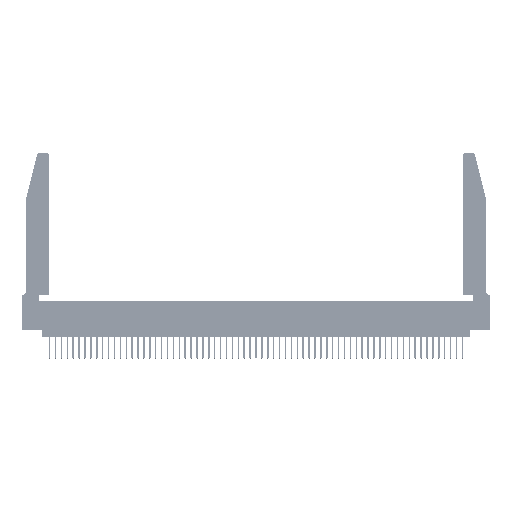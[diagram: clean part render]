
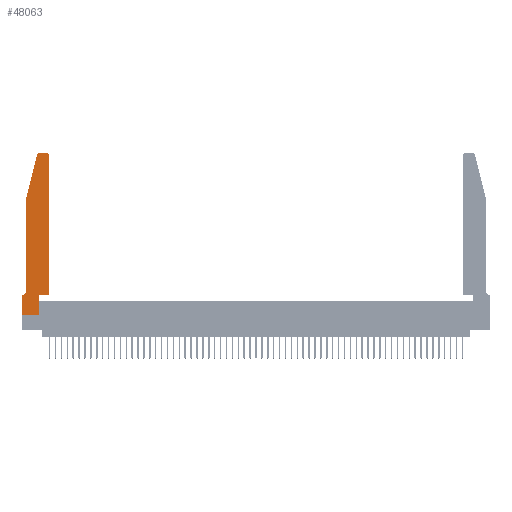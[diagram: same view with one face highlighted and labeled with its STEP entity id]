
A CAD part, top view. The second image highlights one B-rep face of the part: STEP entity #48063.
In plain terms, the highlighted planar face has unit normal (0, 0, 1).
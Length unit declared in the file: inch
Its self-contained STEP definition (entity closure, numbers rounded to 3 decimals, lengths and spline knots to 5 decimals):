
#172 = DIRECTION ( 'NONE',  ( 1., 0., 0. ) ) ;
#823 = ORIENTED_EDGE ( 'NONE', *, *, #5910, .T. ) ;
#1423 = CARTESIAN_POINT ( 'NONE',  ( 0.25487, 2.72718, 0.37 ) ) ;
#2448 = EDGE_CURVE ( 'NONE', #18246, #47984, #6091, .T. ) ;
#2559 = VECTOR ( 'NONE', #38173, 39.37008 ) ;
#2730 = EDGE_CURVE ( 'NONE', #42334, #43385, #30705, .T. ) ;
#3344 = EDGE_CURVE ( 'NONE', #19244, #55225, #32677, .T. ) ;
#3789 = VERTEX_POINT ( 'NONE', #31231 ) ;
#3882 = AXIS2_PLACEMENT_3D ( 'NONE', #48241, #13172, #172 ) ;
#4215 = ORIENTED_EDGE ( 'NONE', *, *, #23464, .T. ) ;
#4382 = DIRECTION ( 'NONE',  ( 0., 0., -1. ) ) ;
#4661 = VECTOR ( 'NONE', #14905, 39.37008 ) ;
#5910 = EDGE_CURVE ( 'NONE', #47984, #21280, #13025, .T. ) ;
#6091 = CIRCLE ( 'NONE', #30854, 0.07 ) ;
#6261 = CARTESIAN_POINT ( 'NONE',  ( 0.2605, 2.75, 0.37 ) ) ;
#6502 = EDGE_CURVE ( 'NONE', #21280, #49266, #38281, .T. ) ;
#8164 = ORIENTED_EDGE ( 'NONE', *, *, #10751, .T. ) ;
#8358 = EDGE_CURVE ( 'NONE', #3789, #42334, #39442, .T. ) ;
#8872 = CIRCLE ( 'NONE', #41871, 0.03 ) ;
#10426 = DIRECTION ( 'NONE',  ( 1., 0., 0. ) ) ;
#10751 = EDGE_CURVE ( 'NONE', #31070, #50438, #34426, .T. ) ;
#11886 = EDGE_CURVE ( 'NONE', #55225, #18246, #43211, .T. ) ;
#12282 = VECTOR ( 'NONE', #23956, 39.37008 ) ;
#12892 = CARTESIAN_POINT ( 'NONE',  ( 0.4205, 2.75, 0.37 ) ) ;
#13025 = LINE ( 'NONE', #19317, #48724 ) ;
#13061 = CARTESIAN_POINT ( 'NONE',  ( 0.4505, 0.35, 0.37 ) ) ;
#13172 = DIRECTION ( 'NONE',  ( 0., 0., 1. ) ) ;
#13239 = EDGE_CURVE ( 'NONE', #43385, #19244, #8872, .T. ) ;
#13485 = EDGE_CURVE ( 'NONE', #50438, #21127, #14307, .T. ) ;
#13586 = CARTESIAN_POINT ( 'NONE',  ( 0.0055, 0.42, 0.37 ) ) ;
#14307 = LINE ( 'NONE', #41436, #12282 ) ;
#14905 = DIRECTION ( 'NONE',  ( -1., 0., 0. ) ) ;
#15164 = VECTOR ( 'NONE', #35005, 39.37008 ) ;
#17438 = DIRECTION ( 'NONE',  ( 0., 1., 0. ) ) ;
#18246 = VERTEX_POINT ( 'NONE', #23071 ) ;
#18422 = LINE ( 'NONE', #13061, #56195 ) ;
#18493 = CARTESIAN_POINT ( 'NONE',  ( 0., 0., 0.37 ) ) ;
#19183 = CARTESIAN_POINT ( 'NONE',  ( 0., 0.35, 0.37 ) ) ;
#19244 = VERTEX_POINT ( 'NONE', #1423 ) ;
#19317 = CARTESIAN_POINT ( 'NONE',  ( 0.0755, 0.35, 0.37 ) ) ;
#20420 = CARTESIAN_POINT ( 'NONE',  ( 0.2865, 0.35, 0.37 ) ) ;
#21127 = VERTEX_POINT ( 'NONE', #27607 ) ;
#21280 = VERTEX_POINT ( 'NONE', #19183 ) ;
#21567 = PLANE ( 'NONE',  #3882 ) ;
#23071 = CARTESIAN_POINT ( 'NONE',  ( 0.0755, 0.42, 0.37 ) ) ;
#23464 = EDGE_CURVE ( 'NONE', #49266, #31070, #41854, .T. ) ;
#23956 = DIRECTION ( 'NONE',  ( 1., 0., 0. ) ) ;
#24555 = FACE_OUTER_BOUND ( 'NONE', #56241, .T. ) ;
#25381 = DIRECTION ( 'NONE',  ( 0., 0., 1. ) ) ;
#27044 = ORIENTED_EDGE ( 'NONE', *, *, #13239, .T. ) ;
#27241 = CARTESIAN_POINT ( 'NONE',  ( 0.284, 2.72, 0.37 ) ) ;
#27306 = CARTESIAN_POINT ( 'NONE',  ( 0.0755, 2., 0.37 ) ) ;
#27607 = CARTESIAN_POINT ( 'NONE',  ( 0.4505, 0.35, 0.37 ) ) ;
#28057 = ORIENTED_EDGE ( 'NONE', *, *, #13485, .T. ) ;
#28301 = ORIENTED_EDGE ( 'NONE', *, *, #3344, .T. ) ;
#28342 = ORIENTED_EDGE ( 'NONE', *, *, #6502, .T. ) ;
#28795 = ORIENTED_EDGE ( 'NONE', *, *, #8358, .T. ) ;
#29490 = CARTESIAN_POINT ( 'NONE',  ( 0., 0., 0.37 ) ) ;
#30705 = LINE ( 'NONE', #6261, #4661 ) ;
#30802 = DIRECTION ( 'NONE',  ( -1., 0., 0. ) ) ;
#30854 = AXIS2_PLACEMENT_3D ( 'NONE', #13586, #4382, #30802 ) ;
#31070 = VERTEX_POINT ( 'NONE', #52534 ) ;
#31231 = CARTESIAN_POINT ( 'NONE',  ( 0.4505, 2.72, 0.37 ) ) ;
#31461 = AXIS2_PLACEMENT_3D ( 'NONE', #52076, #25381, #34208 ) ;
#32157 = DIRECTION ( 'NONE',  ( -1., 0., 0. ) ) ;
#32677 = LINE ( 'NONE', #42022, #2559 ) ;
#32907 = CARTESIAN_POINT ( 'NONE',  ( 0.284, 2.75, 0.37 ) ) ;
#33940 = ORIENTED_EDGE ( 'NONE', *, *, #11886, .T. ) ;
#34208 = DIRECTION ( 'NONE',  ( 1., 0., 0. ) ) ;
#34426 = LINE ( 'NONE', #20420, #54399 ) ;
#35005 = DIRECTION ( 'NONE',  ( 1., 0., 0. ) ) ;
#35408 = EDGE_CURVE ( 'NONE', #21127, #3789, #18422, .T. ) ;
#38173 = DIRECTION ( 'NONE',  ( -0.239, -0.971, 0. ) ) ;
#38281 = LINE ( 'NONE', #18493, #42411 ) ;
#39442 = CIRCLE ( 'NONE', #31461, 0.03 ) ;
#41436 = CARTESIAN_POINT ( 'NONE',  ( 0.4505, 0.35, 0.37 ) ) ;
#41854 = LINE ( 'NONE', #47936, #15164 ) ;
#41871 = AXIS2_PLACEMENT_3D ( 'NONE', #27241, #44890, #10426 ) ;
#42022 = CARTESIAN_POINT ( 'NONE',  ( 0.0755, 2., 0.37 ) ) ;
#42334 = VERTEX_POINT ( 'NONE', #12892 ) ;
#42411 = VECTOR ( 'NONE', #49203, 39.37008 ) ;
#43211 = LINE ( 'NONE', #51362, #43919 ) ;
#43385 = VERTEX_POINT ( 'NONE', #32907 ) ;
#43919 = VECTOR ( 'NONE', #46941, 39.37008 ) ;
#44890 = DIRECTION ( 'NONE',  ( 0., 0., 1. ) ) ;
#46941 = DIRECTION ( 'NONE',  ( 0., -1., 0. ) ) ;
#47936 = CARTESIAN_POINT ( 'NONE',  ( 0., 0., 0.37 ) ) ;
#47984 = VERTEX_POINT ( 'NONE', #51532 ) ;
#48063 = ADVANCED_FACE ( 'NONE', ( #24555 ), #21567, .T. ) ;
#48241 = CARTESIAN_POINT ( 'NONE',  ( 0., 0.35, 0.37 ) ) ;
#48724 = VECTOR ( 'NONE', #32157, 39.37008 ) ;
#49203 = DIRECTION ( 'NONE',  ( 0., -1., 0. ) ) ;
#49266 = VERTEX_POINT ( 'NONE', #29490 ) ;
#49295 = ORIENTED_EDGE ( 'NONE', *, *, #35408, .T. ) ;
#50438 = VERTEX_POINT ( 'NONE', #52351 ) ;
#51362 = CARTESIAN_POINT ( 'NONE',  ( 0.0755, 2., 0.37 ) ) ;
#51532 = CARTESIAN_POINT ( 'NONE',  ( 0.0055, 0.35, 0.37 ) ) ;
#52046 = DIRECTION ( 'NONE',  ( 0., 1., 0. ) ) ;
#52076 = CARTESIAN_POINT ( 'NONE',  ( 0.4205, 2.72, 0.37 ) ) ;
#52351 = CARTESIAN_POINT ( 'NONE',  ( 0.2865, 0.35, 0.37 ) ) ;
#52534 = CARTESIAN_POINT ( 'NONE',  ( 0.2865, 0., 0.37 ) ) ;
#53919 = ORIENTED_EDGE ( 'NONE', *, *, #2448, .T. ) ;
#54399 = VECTOR ( 'NONE', #52046, 39.37008 ) ;
#55225 = VERTEX_POINT ( 'NONE', #27306 ) ;
#55352 = ORIENTED_EDGE ( 'NONE', *, *, #2730, .T. ) ;
#56195 = VECTOR ( 'NONE', #17438, 39.37008 ) ;
#56241 = EDGE_LOOP ( 'NONE', ( #55352, #27044, #28301, #33940, #53919, #823, #28342, #4215, #8164, #28057, #49295, #28795 ) ) ;
